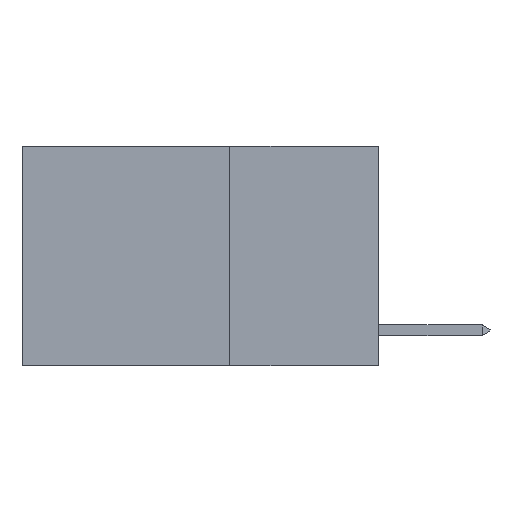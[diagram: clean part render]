
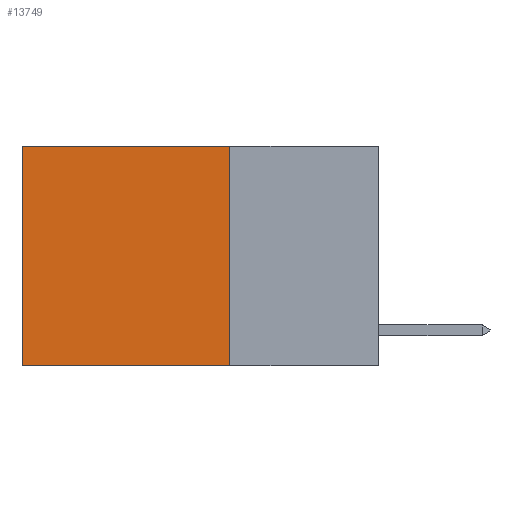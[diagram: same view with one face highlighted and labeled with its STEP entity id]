
A CAD part, left-side view. The second image highlights one B-rep face of the part: STEP entity #13749.
In plain terms, the highlighted planar face has unit normal (-1, 0, 0).
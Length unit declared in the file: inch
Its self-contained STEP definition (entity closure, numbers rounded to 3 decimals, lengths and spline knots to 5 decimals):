
#95 = ORIENTED_EDGE ( 'NONE', *, *, #4072, .F. ) ;
#1664 = LINE ( 'NONE', #11357, #11160 ) ;
#1845 = LINE ( 'NONE', #22791, #7480 ) ;
#1900 = EDGE_CURVE ( 'NONE', #2089, #2495, #1664, .T. ) ;
#2089 = VERTEX_POINT ( 'NONE', #19497 ) ;
#2495 = VERTEX_POINT ( 'NONE', #14857 ) ;
#3092 = VECTOR ( 'NONE', #20890, 39.37008 ) ;
#3353 = CARTESIAN_POINT ( 'NONE',  ( 0.2625, 0.6, -0.37 ) ) ;
#3600 = DIRECTION ( 'NONE',  ( 0., 1., 0. ) ) ;
#3788 = DIRECTION ( 'NONE',  ( 0., 0., -1. ) ) ;
#3908 = CARTESIAN_POINT ( 'NONE',  ( 0.2625, 0.6, 0. ) ) ;
#4072 = EDGE_CURVE ( 'NONE', #2495, #17599, #1845, .T. ) ;
#5454 = ORIENTED_EDGE ( 'NONE', *, *, #21014, .T. ) ;
#5703 = CARTESIAN_POINT ( 'NONE',  ( 0.2625, 0.25, 0. ) ) ;
#7480 = VECTOR ( 'NONE', #19338, 39.37008 ) ;
#7620 = DIRECTION ( 'NONE',  ( 1., 0., 0. ) ) ;
#7868 = CARTESIAN_POINT ( 'NONE',  ( 0.2625, 0.6, 0. ) ) ;
#8395 = ORIENTED_EDGE ( 'NONE', *, *, #15817, .T. ) ;
#8551 = AXIS2_PLACEMENT_3D ( 'NONE', #5703, #7620, #20795 ) ;
#8730 = LINE ( 'NONE', #3908, #3092 ) ;
#8844 = LINE ( 'NONE', #20542, #22563 ) ;
#9744 = VERTEX_POINT ( 'NONE', #7868 ) ;
#11160 = VECTOR ( 'NONE', #3788, 39.37008 ) ;
#11357 = CARTESIAN_POINT ( 'NONE',  ( 0.2625, 0.25, 0. ) ) ;
#11374 = PLANE ( 'NONE',  #8551 ) ;
#13749 = ADVANCED_FACE ( 'NONE', ( #23798 ), #11374, .F. ) ;
#14857 = CARTESIAN_POINT ( 'NONE',  ( 0.2625, 0.25, -0.37 ) ) ;
#15817 = EDGE_CURVE ( 'NONE', #2089, #9744, #8844, .T. ) ;
#17599 = VERTEX_POINT ( 'NONE', #3353 ) ;
#17900 = ORIENTED_EDGE ( 'NONE', *, *, #1900, .F. ) ;
#19338 = DIRECTION ( 'NONE',  ( 0., 1., 0. ) ) ;
#19497 = CARTESIAN_POINT ( 'NONE',  ( 0.2625, 0.25, 0. ) ) ;
#20542 = CARTESIAN_POINT ( 'NONE',  ( 0.2625, 0.25, 0. ) ) ;
#20795 = DIRECTION ( 'NONE',  ( 0., 0., -1. ) ) ;
#20890 = DIRECTION ( 'NONE',  ( 0., 0., -1. ) ) ;
#21014 = EDGE_CURVE ( 'NONE', #9744, #17599, #8730, .T. ) ;
#22563 = VECTOR ( 'NONE', #3600, 39.37008 ) ;
#22791 = CARTESIAN_POINT ( 'NONE',  ( 0.2625, 0.25, -0.37 ) ) ;
#23190 = EDGE_LOOP ( 'NONE', ( #5454, #95, #17900, #8395 ) ) ;
#23798 = FACE_OUTER_BOUND ( 'NONE', #23190, .T. ) ;
